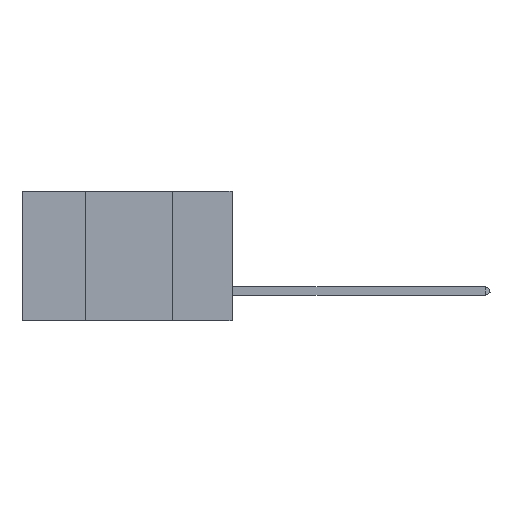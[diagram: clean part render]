
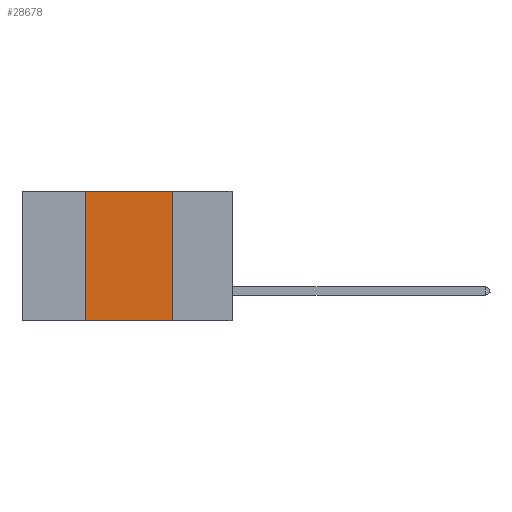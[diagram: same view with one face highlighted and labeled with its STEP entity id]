
A CAD part, left-side view. The second image highlights one B-rep face of the part: STEP entity #28678.
In plain terms, the highlighted planar face has unit normal (-1, 0, 0).
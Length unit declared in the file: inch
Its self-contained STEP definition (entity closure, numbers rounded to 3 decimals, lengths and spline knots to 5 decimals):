
#604 = CARTESIAN_POINT ( 'NONE',  ( 0., 0.17, 0. ) ) ;
#1093 = VECTOR ( 'NONE', #4652, 39.37008 ) ;
#1113 = CARTESIAN_POINT ( 'NONE',  ( 0., 0.42, -0.37 ) ) ;
#1964 = VERTEX_POINT ( 'NONE', #23433 ) ;
#2113 = LINE ( 'NONE', #9684, #1093 ) ;
#2397 = CARTESIAN_POINT ( 'NONE',  ( 0., 0.6, 0. ) ) ;
#2741 = VECTOR ( 'NONE', #28137, 39.37008 ) ;
#4652 = DIRECTION ( 'NONE',  ( 0., -1., 0. ) ) ;
#5492 = LINE ( 'NONE', #21381, #2741 ) ;
#5903 = VECTOR ( 'NONE', #10320, 39.37008 ) ;
#6615 = EDGE_CURVE ( 'NONE', #14784, #1964, #5492, .T. ) ;
#7032 = DIRECTION ( 'NONE',  ( 0., -1., 0. ) ) ;
#8681 = ORIENTED_EDGE ( 'NONE', *, *, #27088, .F. ) ;
#9684 = CARTESIAN_POINT ( 'NONE',  ( 0., 0.6, -0.37 ) ) ;
#10320 = DIRECTION ( 'NONE',  ( 0., 0., 1. ) ) ;
#10579 = DIRECTION ( 'NONE',  ( 0., 0., -1. ) ) ;
#11869 = VERTEX_POINT ( 'NONE', #16288 ) ;
#14490 = CARTESIAN_POINT ( 'NONE',  ( 0., 0.42, 0. ) ) ;
#14784 = VERTEX_POINT ( 'NONE', #604 ) ;
#15017 = VECTOR ( 'NONE', #7032, 39.37008 ) ;
#15507 = AXIS2_PLACEMENT_3D ( 'NONE', #21691, #19069, #10579 ) ;
#16013 = EDGE_CURVE ( 'NONE', #25577, #11869, #21514, .T. ) ;
#16214 = ORIENTED_EDGE ( 'NONE', *, *, #16013, .F. ) ;
#16288 = CARTESIAN_POINT ( 'NONE',  ( 0., 0.42, 0. ) ) ;
#19069 = DIRECTION ( 'NONE',  ( 1., 0., 0. ) ) ;
#19844 = EDGE_CURVE ( 'NONE', #25577, #1964, #2113, .T. ) ;
#20542 = EDGE_LOOP ( 'NONE', ( #22975, #8681, #16214, #21966 ) ) ;
#21381 = CARTESIAN_POINT ( 'NONE',  ( 0., 0.17, 0. ) ) ;
#21514 = LINE ( 'NONE', #14490, #5903 ) ;
#21691 = CARTESIAN_POINT ( 'NONE',  ( 0., 0.6, 0. ) ) ;
#21908 = LINE ( 'NONE', #2397, #15017 ) ;
#21966 = ORIENTED_EDGE ( 'NONE', *, *, #19844, .T. ) ;
#22975 = ORIENTED_EDGE ( 'NONE', *, *, #6615, .F. ) ;
#23433 = CARTESIAN_POINT ( 'NONE',  ( 0., 0.17, -0.37 ) ) ;
#25577 = VERTEX_POINT ( 'NONE', #1113 ) ;
#25863 = PLANE ( 'NONE',  #15507 ) ;
#27088 = EDGE_CURVE ( 'NONE', #11869, #14784, #21908, .T. ) ;
#28137 = DIRECTION ( 'NONE',  ( 0., 0., -1. ) ) ;
#28365 = FACE_OUTER_BOUND ( 'NONE', #20542, .T. ) ;
#28678 = ADVANCED_FACE ( 'NONE', ( #28365 ), #25863, .F. ) ;
